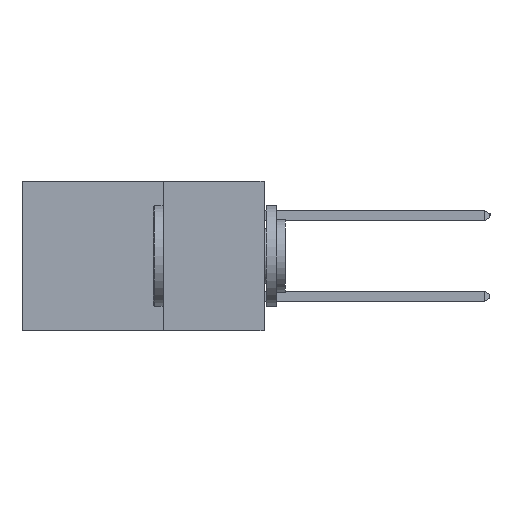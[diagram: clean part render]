
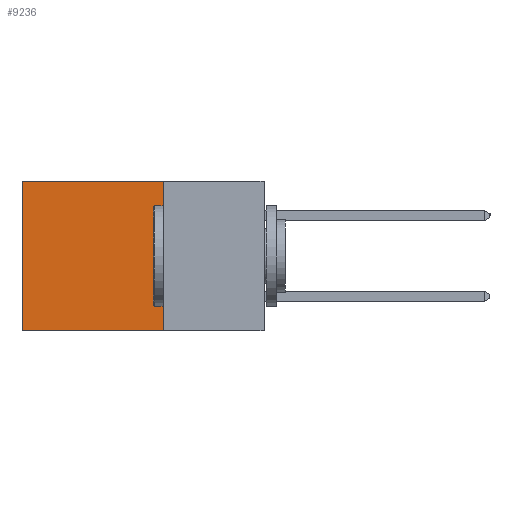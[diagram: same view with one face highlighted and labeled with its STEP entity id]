
A CAD part, left-side view. The second image highlights one B-rep face of the part: STEP entity #9236.
In plain terms, the highlighted planar face has unit normal (-1, 0, 0).
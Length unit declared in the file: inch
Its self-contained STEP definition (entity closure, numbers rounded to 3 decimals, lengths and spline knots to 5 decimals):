
#878 = DIRECTION ( 'NONE',  ( 0., 1., 0. ) ) ;
#881 = VERTEX_POINT ( 'NONE', #16014 ) ;
#2565 = EDGE_CURVE ( 'NONE', #6454, #4710, #8270, .T. ) ;
#3327 = CARTESIAN_POINT ( 'NONE',  ( 0.2615, 0.25, -0.37 ) ) ;
#4710 = VERTEX_POINT ( 'NONE', #6752 ) ;
#4887 = EDGE_LOOP ( 'NONE', ( #10545, #14779, #7770, #16189 ) ) ;
#5144 = DIRECTION ( 'NONE',  ( 0., 0., -1. ) ) ;
#5160 = CARTESIAN_POINT ( 'NONE',  ( 0.2615, 0.25, 0. ) ) ;
#5205 = DIRECTION ( 'NONE',  ( 1., 0., 0. ) ) ;
#5309 = DIRECTION ( 'NONE',  ( 0., 0., -1. ) ) ;
#5408 = PLANE ( 'NONE',  #17781 ) ;
#5478 = DIRECTION ( 'NONE',  ( 0., 0., -1. ) ) ;
#6454 = VERTEX_POINT ( 'NONE', #5160 ) ;
#6752 = CARTESIAN_POINT ( 'NONE',  ( 0.2615, 0.25, -0.37 ) ) ;
#7347 = CARTESIAN_POINT ( 'NONE',  ( 0.2615, 0.25, 0. ) ) ;
#7770 = ORIENTED_EDGE ( 'NONE', *, *, #2565, .F. ) ;
#7963 = EDGE_CURVE ( 'NONE', #6454, #11242, #12018, .T. ) ;
#8270 = LINE ( 'NONE', #19359, #12661 ) ;
#9236 = ADVANCED_FACE ( 'NONE', ( #13197 ), #5408, .F. ) ;
#9537 = CARTESIAN_POINT ( 'NONE',  ( 0.2615, 0.6, 0. ) ) ;
#9820 = VECTOR ( 'NONE', #878, 39.37008 ) ;
#10545 = ORIENTED_EDGE ( 'NONE', *, *, #12894, .T. ) ;
#10900 = VECTOR ( 'NONE', #13716, 39.37008 ) ;
#11242 = VERTEX_POINT ( 'NONE', #9537 ) ;
#11729 = LINE ( 'NONE', #18039, #19502 ) ;
#11768 = LINE ( 'NONE', #15478, #10900 ) ;
#12018 = LINE ( 'NONE', #7347, #9820 ) ;
#12647 = EDGE_CURVE ( 'NONE', #4710, #881, #11768, .T. ) ;
#12661 = VECTOR ( 'NONE', #5144, 39.37008 ) ;
#12894 = EDGE_CURVE ( 'NONE', #11242, #881, #11729, .T. ) ;
#13197 = FACE_OUTER_BOUND ( 'NONE', #4887, .T. ) ;
#13716 = DIRECTION ( 'NONE',  ( 0., 1., 0. ) ) ;
#14779 = ORIENTED_EDGE ( 'NONE', *, *, #12647, .F. ) ;
#15478 = CARTESIAN_POINT ( 'NONE',  ( 0.2615, 0.25, -0.37 ) ) ;
#16014 = CARTESIAN_POINT ( 'NONE',  ( 0.2615, 0.6, -0.37 ) ) ;
#16189 = ORIENTED_EDGE ( 'NONE', *, *, #7963, .T. ) ;
#17781 = AXIS2_PLACEMENT_3D ( 'NONE', #3327, #5205, #5309 ) ;
#18039 = CARTESIAN_POINT ( 'NONE',  ( 0.2615, 0.6, -0.37 ) ) ;
#19359 = CARTESIAN_POINT ( 'NONE',  ( 0.2615, 0.25, -0.37 ) ) ;
#19502 = VECTOR ( 'NONE', #5478, 39.37008 ) ;
